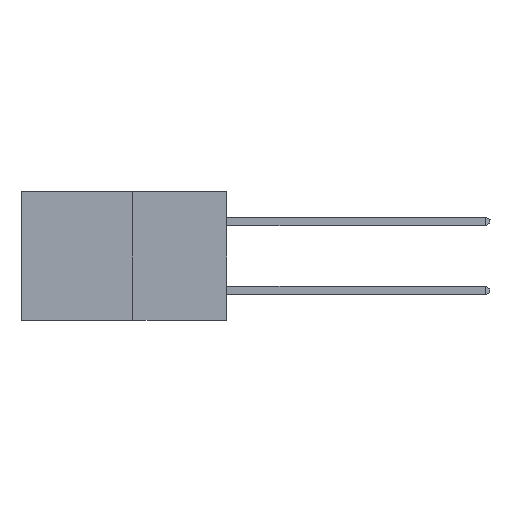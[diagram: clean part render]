
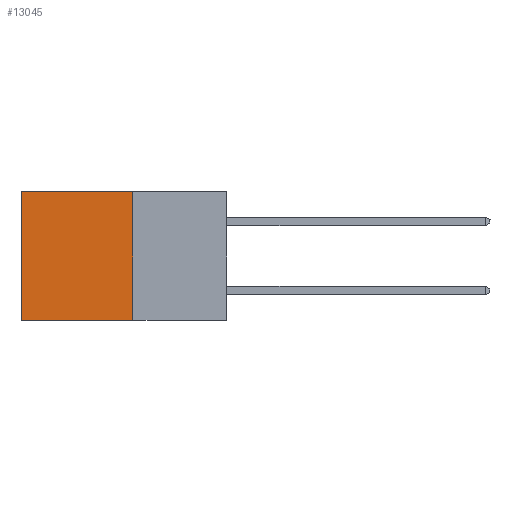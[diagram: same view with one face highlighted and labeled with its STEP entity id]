
A CAD part, left-side view. The second image highlights one B-rep face of the part: STEP entity #13045.
In plain terms, the highlighted planar face has unit normal (-1, 0, 0).
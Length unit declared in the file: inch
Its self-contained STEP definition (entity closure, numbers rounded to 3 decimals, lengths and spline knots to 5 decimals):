
#808 = EDGE_CURVE ( 'NONE', #23794, #22723, #8184, .T. ) ;
#2359 = CARTESIAN_POINT ( 'NONE',  ( 0.277, 0.59, -0.37 ) ) ;
#3947 = ORIENTED_EDGE ( 'NONE', *, *, #808, .T. ) ;
#4084 = DIRECTION ( 'NONE',  ( 0., 1., 0. ) ) ;
#7100 = CARTESIAN_POINT ( 'NONE',  ( 0.277, 0.27, -0.37 ) ) ;
#8138 = EDGE_LOOP ( 'NONE', ( #3947, #26203, #10594, #11226 ) ) ;
#8184 = LINE ( 'NONE', #23605, #23705 ) ;
#8690 = FACE_OUTER_BOUND ( 'NONE', #8138, .T. ) ;
#9922 = CARTESIAN_POINT ( 'NONE',  ( 0.277, 0.59, 0. ) ) ;
#10190 = VERTEX_POINT ( 'NONE', #22793 ) ;
#10594 = ORIENTED_EDGE ( 'NONE', *, *, #21207, .F. ) ;
#11162 = DIRECTION ( 'NONE',  ( 0., 0., -1. ) ) ;
#11226 = ORIENTED_EDGE ( 'NONE', *, *, #16553, .T. ) ;
#11768 = DIRECTION ( 'NONE',  ( 0., 0., -1. ) ) ;
#12617 = LINE ( 'NONE', #23477, #23428 ) ;
#13045 = ADVANCED_FACE ( 'NONE', ( #8690 ), #21229, .F. ) ;
#13128 = CARTESIAN_POINT ( 'NONE',  ( 0.277, 0.27, 0. ) ) ;
#13340 = DIRECTION ( 'NONE',  ( 0., 1., 0. ) ) ;
#13929 = VECTOR ( 'NONE', #4084, 39.37008 ) ;
#14326 = VERTEX_POINT ( 'NONE', #13128 ) ;
#16144 = EDGE_CURVE ( 'NONE', #10190, #22723, #22808, .T. ) ;
#16553 = EDGE_CURVE ( 'NONE', #14326, #23794, #12617, .T. ) ;
#17135 = DIRECTION ( 'NONE',  ( 0., 0., -1. ) ) ;
#17149 = CARTESIAN_POINT ( 'NONE',  ( 0.277, 0.27, -0.37 ) ) ;
#18195 = CARTESIAN_POINT ( 'NONE',  ( 0.277, 0.27, -0.37 ) ) ;
#18263 = LINE ( 'NONE', #7100, #18913 ) ;
#18913 = VECTOR ( 'NONE', #17135, 39.37008 ) ;
#21207 = EDGE_CURVE ( 'NONE', #14326, #10190, #18263, .T. ) ;
#21229 = PLANE ( 'NONE',  #22945 ) ;
#22723 = VERTEX_POINT ( 'NONE', #2359 ) ;
#22793 = CARTESIAN_POINT ( 'NONE',  ( 0.277, 0.27, -0.37 ) ) ;
#22808 = LINE ( 'NONE', #18195, #13929 ) ;
#22945 = AXIS2_PLACEMENT_3D ( 'NONE', #17149, #23313, #11162 ) ;
#23313 = DIRECTION ( 'NONE',  ( 1., 0., 0. ) ) ;
#23428 = VECTOR ( 'NONE', #13340, 39.37008 ) ;
#23477 = CARTESIAN_POINT ( 'NONE',  ( 0.277, 0.27, 0. ) ) ;
#23605 = CARTESIAN_POINT ( 'NONE',  ( 0.277, 0.59, -0.37 ) ) ;
#23705 = VECTOR ( 'NONE', #11768, 39.37008 ) ;
#23794 = VERTEX_POINT ( 'NONE', #9922 ) ;
#26203 = ORIENTED_EDGE ( 'NONE', *, *, #16144, .F. ) ;
